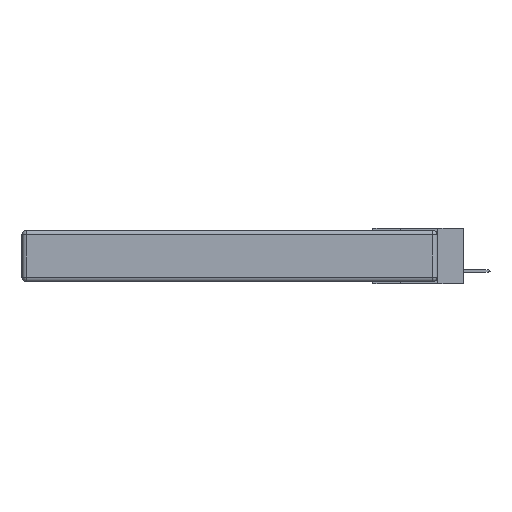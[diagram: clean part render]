
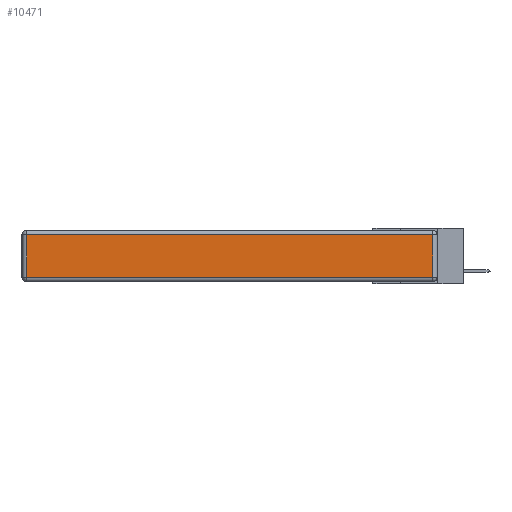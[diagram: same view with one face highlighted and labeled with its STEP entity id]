
A CAD part, left-side view. The second image highlights one B-rep face of the part: STEP entity #10471.
In plain terms, the highlighted planar face has unit normal (-1, 0, 0).
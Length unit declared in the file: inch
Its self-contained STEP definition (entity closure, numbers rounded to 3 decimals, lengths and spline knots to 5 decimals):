
#770 = VERTEX_POINT ( 'NONE', #6528 ) ;
#1450 = AXIS2_PLACEMENT_3D ( 'NONE', #8854, #3615, #10234 ) ;
#1760 = CARTESIAN_POINT ( 'NONE',  ( 0., 0., -0.313 ) ) ;
#2790 = EDGE_CURVE ( 'NONE', #5555, #3976, #4965, .T. ) ;
#3169 = DIRECTION ( 'NONE',  ( 0., -1., 0. ) ) ;
#3330 = LINE ( 'NONE', #16305, #11863 ) ;
#3485 = CARTESIAN_POINT ( 'NONE',  ( 0., 2.72, -0.313 ) ) ;
#3615 = DIRECTION ( 'NONE',  ( -1., 0., 0. ) ) ;
#3976 = VERTEX_POINT ( 'NONE', #14854 ) ;
#4333 = CARTESIAN_POINT ( 'NONE',  ( 0., 0.03, -0.03 ) ) ;
#4896 = EDGE_LOOP ( 'NONE', ( #9153, #6608, #7298, #7610 ) ) ;
#4965 = LINE ( 'NONE', #1760, #9670 ) ;
#5258 = DIRECTION ( 'NONE',  ( 0., 0., 1. ) ) ;
#5472 = EDGE_CURVE ( 'NONE', #10215, #770, #3330, .T. ) ;
#5555 = VERTEX_POINT ( 'NONE', #3485 ) ;
#6528 = CARTESIAN_POINT ( 'NONE',  ( 0., 2.72, -0.03 ) ) ;
#6608 = ORIENTED_EDGE ( 'NONE', *, *, #16137, .T. ) ;
#7146 = LINE ( 'NONE', #9697, #14130 ) ;
#7298 = ORIENTED_EDGE ( 'NONE', *, *, #5472, .T. ) ;
#7610 = ORIENTED_EDGE ( 'NONE', *, *, #12116, .T. ) ;
#8854 = CARTESIAN_POINT ( 'NONE',  ( 0., 0., -0.343 ) ) ;
#9153 = ORIENTED_EDGE ( 'NONE', *, *, #2790, .T. ) ;
#9541 = DIRECTION ( 'NONE',  ( 0., 1., 0. ) ) ;
#9670 = VECTOR ( 'NONE', #3169, 39.37008 ) ;
#9697 = CARTESIAN_POINT ( 'NONE',  ( 0., 2.72, -0.343 ) ) ;
#10215 = VERTEX_POINT ( 'NONE', #4333 ) ;
#10234 = DIRECTION ( 'NONE',  ( 0., 0., 1. ) ) ;
#10471 = ADVANCED_FACE ( 'NONE', ( #11031 ), #17125, .T. ) ;
#10690 = VECTOR ( 'NONE', #5258, 39.37008 ) ;
#10736 = CARTESIAN_POINT ( 'NONE',  ( 0., 0.03, -0.343 ) ) ;
#11031 = FACE_OUTER_BOUND ( 'NONE', #4896, .T. ) ;
#11863 = VECTOR ( 'NONE', #9541, 39.37008 ) ;
#12116 = EDGE_CURVE ( 'NONE', #770, #5555, #7146, .T. ) ;
#14130 = VECTOR ( 'NONE', #15256, 39.37008 ) ;
#14276 = LINE ( 'NONE', #10736, #10690 ) ;
#14854 = CARTESIAN_POINT ( 'NONE',  ( 0., 0.03, -0.313 ) ) ;
#15256 = DIRECTION ( 'NONE',  ( 0., 0., -1. ) ) ;
#16137 = EDGE_CURVE ( 'NONE', #3976, #10215, #14276, .T. ) ;
#16305 = CARTESIAN_POINT ( 'NONE',  ( 0., 2.75, -0.03 ) ) ;
#17125 = PLANE ( 'NONE',  #1450 ) ;
